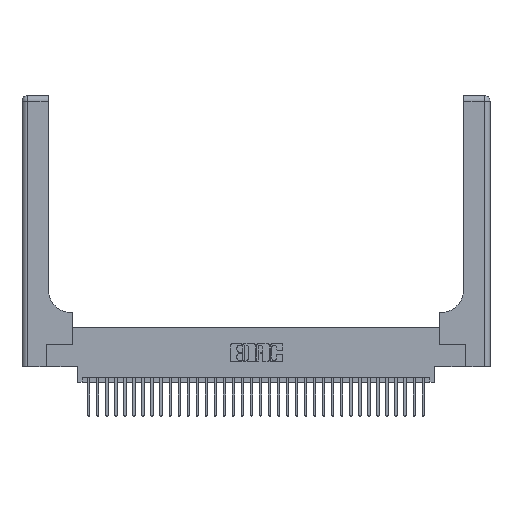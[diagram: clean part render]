
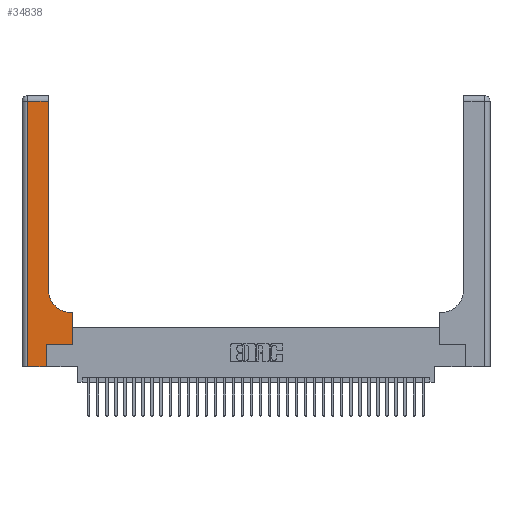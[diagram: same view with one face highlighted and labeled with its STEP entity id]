
A CAD part, top view. The second image highlights one B-rep face of the part: STEP entity #34838.
In plain terms, the highlighted planar face has unit normal (0, 0, 1).
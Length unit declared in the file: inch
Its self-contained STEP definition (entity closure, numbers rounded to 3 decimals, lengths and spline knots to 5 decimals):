
#738 = EDGE_CURVE ( 'NONE', #8885, #32104, #14489, .T. ) ;
#939 = CARTESIAN_POINT ( 'NONE',  ( 0., 2.94, 0.37 ) ) ;
#1579 = EDGE_CURVE ( 'NONE', #7923, #12202, #17114, .T. ) ;
#3121 = VECTOR ( 'NONE', #24852, 39.37008 ) ;
#3702 = VERTEX_POINT ( 'NONE', #17811 ) ;
#3707 = CARTESIAN_POINT ( 'NONE',  ( 0.2915, 0.6, 0.37 ) ) ;
#3993 = LINE ( 'NONE', #3707, #3121 ) ;
#4460 = DIRECTION ( 'NONE',  ( -1., 0., 0. ) ) ;
#4800 = CARTESIAN_POINT ( 'NONE',  ( 0.269, 0.25, 0.37 ) ) ;
#4988 = VECTOR ( 'NONE', #22385, 39.37008 ) ;
#6004 = ORIENTED_EDGE ( 'NONE', *, *, #31418, .T. ) ;
#6489 = VERTEX_POINT ( 'NONE', #6695 ) ;
#6695 = CARTESIAN_POINT ( 'NONE',  ( 0.06, 2.94, 0.37 ) ) ;
#7923 = VERTEX_POINT ( 'NONE', #21033 ) ;
#8885 = VERTEX_POINT ( 'NONE', #18595 ) ;
#9523 = LINE ( 'NONE', #4800, #16799 ) ;
#9724 = VERTEX_POINT ( 'NONE', #24885 ) ;
#9799 = EDGE_CURVE ( 'NONE', #21086, #31620, #26936, .T. ) ;
#10718 = CARTESIAN_POINT ( 'NONE',  ( 0.5585, 0.25, 0.37 ) ) ;
#12060 = EDGE_CURVE ( 'NONE', #12202, #9724, #21222, .T. ) ;
#12202 = VERTEX_POINT ( 'NONE', #21103 ) ;
#12831 = AXIS2_PLACEMENT_3D ( 'NONE', #15434, #20992, #4460 ) ;
#12858 = CARTESIAN_POINT ( 'NONE',  ( 0.5415, 0.85, 0.37 ) ) ;
#12881 = ORIENTED_EDGE ( 'NONE', *, *, #12060, .T. ) ;
#13363 = LINE ( 'NONE', #14470, #19853 ) ;
#13635 = VECTOR ( 'NONE', #21397, 39.37008 ) ;
#14188 = CARTESIAN_POINT ( 'NONE',  ( 0.5585, 0.25, 0.37 ) ) ;
#14470 = CARTESIAN_POINT ( 'NONE',  ( 0.06, 3., 0.37 ) ) ;
#14489 = LINE ( 'NONE', #35088, #13635 ) ;
#15040 = ORIENTED_EDGE ( 'NONE', *, *, #9799, .T. ) ;
#15375 = VECTOR ( 'NONE', #27632, 39.37008 ) ;
#15434 = CARTESIAN_POINT ( 'NONE',  ( 0., 3., 0.37 ) ) ;
#15593 = DIRECTION ( 'NONE',  ( 1., 0., 0. ) ) ;
#16726 = ORIENTED_EDGE ( 'NONE', *, *, #17532, .T. ) ;
#16799 = VECTOR ( 'NONE', #26703, 39.37008 ) ;
#16971 = CARTESIAN_POINT ( 'NONE',  ( 0.5585, 0.6, 0.37 ) ) ;
#17114 = LINE ( 'NONE', #24879, #15375 ) ;
#17532 = EDGE_CURVE ( 'NONE', #6489, #7923, #13363, .T. ) ;
#17811 = CARTESIAN_POINT ( 'NONE',  ( 0.5415, 0.6, 0.37 ) ) ;
#18056 = FACE_OUTER_BOUND ( 'NONE', #34733, .T. ) ;
#18222 = PLANE ( 'NONE',  #12831 ) ;
#18482 = ORIENTED_EDGE ( 'NONE', *, *, #1579, .T. ) ;
#18595 = CARTESIAN_POINT ( 'NONE',  ( 0.2915, 0.85, 0.37 ) ) ;
#19045 = LINE ( 'NONE', #939, #26305 ) ;
#19853 = VECTOR ( 'NONE', #25518, 39.37008 ) ;
#20289 = DIRECTION ( 'NONE',  ( -1., 0., 0. ) ) ;
#20992 = DIRECTION ( 'NONE',  ( 0., 0., -1. ) ) ;
#21033 = CARTESIAN_POINT ( 'NONE',  ( 0.06, 0., 0.37 ) ) ;
#21086 = VERTEX_POINT ( 'NONE', #10718 ) ;
#21103 = CARTESIAN_POINT ( 'NONE',  ( 0.269, 0., 0.37 ) ) ;
#21222 = LINE ( 'NONE', #28775, #27645 ) ;
#21397 = DIRECTION ( 'NONE',  ( 0., 1., 0. ) ) ;
#21932 = AXIS2_PLACEMENT_3D ( 'NONE', #12858, #32090, #15593 ) ;
#22345 = ORIENTED_EDGE ( 'NONE', *, *, #30628, .T. ) ;
#22385 = DIRECTION ( 'NONE',  ( 0., 1., 0. ) ) ;
#22999 = ORIENTED_EDGE ( 'NONE', *, *, #738, .T. ) ;
#24001 = EDGE_CURVE ( 'NONE', #31620, #3702, #3993, .T. ) ;
#24624 = CIRCLE ( 'NONE', #21932, 0.25 ) ;
#24852 = DIRECTION ( 'NONE',  ( -1., 0., 0. ) ) ;
#24879 = CARTESIAN_POINT ( 'NONE',  ( 0., 0., 0.37 ) ) ;
#24885 = CARTESIAN_POINT ( 'NONE',  ( 0.269, 0.25, 0.37 ) ) ;
#25381 = ORIENTED_EDGE ( 'NONE', *, *, #24001, .T. ) ;
#25518 = DIRECTION ( 'NONE',  ( 0., -1., 0. ) ) ;
#26006 = DIRECTION ( 'NONE',  ( 0., 1., 0. ) ) ;
#26305 = VECTOR ( 'NONE', #20289, 39.37008 ) ;
#26703 = DIRECTION ( 'NONE',  ( 1., 0., 0. ) ) ;
#26936 = LINE ( 'NONE', #14188, #4988 ) ;
#27632 = DIRECTION ( 'NONE',  ( 1., 0., 0. ) ) ;
#27645 = VECTOR ( 'NONE', #26006, 39.37008 ) ;
#28775 = CARTESIAN_POINT ( 'NONE',  ( 0.269, 0., 0.37 ) ) ;
#30227 = EDGE_CURVE ( 'NONE', #3702, #8885, #24624, .T. ) ;
#30628 = EDGE_CURVE ( 'NONE', #32104, #6489, #19045, .T. ) ;
#31418 = EDGE_CURVE ( 'NONE', #9724, #21086, #9523, .T. ) ;
#31620 = VERTEX_POINT ( 'NONE', #16971 ) ;
#32090 = DIRECTION ( 'NONE',  ( 0., 0., -1. ) ) ;
#32104 = VERTEX_POINT ( 'NONE', #32693 ) ;
#32292 = ORIENTED_EDGE ( 'NONE', *, *, #30227, .T. ) ;
#32693 = CARTESIAN_POINT ( 'NONE',  ( 0.2915, 2.94, 0.37 ) ) ;
#34733 = EDGE_LOOP ( 'NONE', ( #22999, #22345, #16726, #18482, #12881, #6004, #15040, #25381, #32292 ) ) ;
#34838 = ADVANCED_FACE ( 'NONE', ( #18056 ), #18222, .F. ) ;
#35088 = CARTESIAN_POINT ( 'NONE',  ( 0.2915, 3., 0.37 ) ) ;
